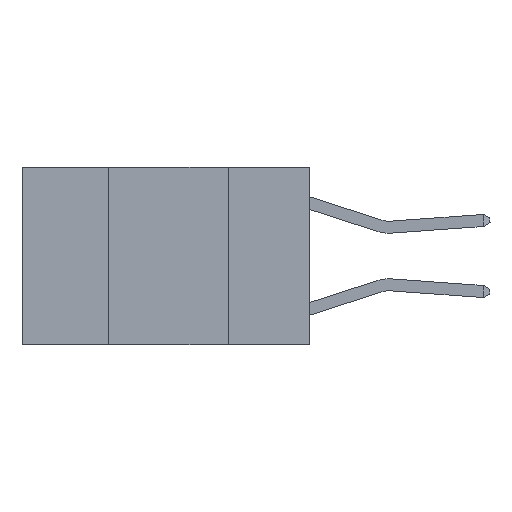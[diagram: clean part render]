
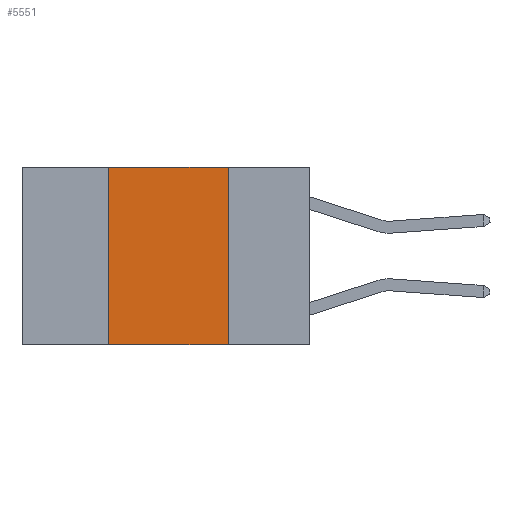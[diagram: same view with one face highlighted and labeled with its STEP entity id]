
A CAD part, left-side view. The second image highlights one B-rep face of the part: STEP entity #5551.
In plain terms, the highlighted planar face has unit normal (-1, 0, 0).
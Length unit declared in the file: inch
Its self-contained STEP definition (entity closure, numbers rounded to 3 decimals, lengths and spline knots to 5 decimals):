
#1247 = FACE_OUTER_BOUND ( 'NONE', #9727, .T. ) ;
#1549 = VERTEX_POINT ( 'NONE', #8327 ) ;
#1572 = CARTESIAN_POINT ( 'NONE',  ( 0., 0.6, 0. ) ) ;
#1805 = CARTESIAN_POINT ( 'NONE',  ( 0., 0.17, 0. ) ) ;
#2002 = CARTESIAN_POINT ( 'NONE',  ( 0., 0.6, 0. ) ) ;
#2233 = VECTOR ( 'NONE', #9315, 39.37008 ) ;
#2656 = DIRECTION ( 'NONE',  ( 0., -1., 0. ) ) ;
#2933 = EDGE_CURVE ( 'NONE', #13584, #8344, #10100, .T. ) ;
#3110 = DIRECTION ( 'NONE',  ( 0., 0., -1. ) ) ;
#3391 = DIRECTION ( 'NONE',  ( 0., 0., 1. ) ) ;
#3417 = ORIENTED_EDGE ( 'NONE', *, *, #9958, .F. ) ;
#3783 = VECTOR ( 'NONE', #3391, 39.37008 ) ;
#4291 = VECTOR ( 'NONE', #3110, 39.37008 ) ;
#4315 = VECTOR ( 'NONE', #2656, 39.37008 ) ;
#4911 = VERTEX_POINT ( 'NONE', #13449 ) ;
#5147 = ORIENTED_EDGE ( 'NONE', *, *, #2933, .F. ) ;
#5224 = EDGE_CURVE ( 'NONE', #1549, #4911, #11999, .T. ) ;
#5268 = PLANE ( 'NONE',  #9720 ) ;
#5498 = EDGE_CURVE ( 'NONE', #1549, #8344, #8744, .T. ) ;
#5551 = ADVANCED_FACE ( 'NONE', ( #1247 ), #5268, .F. ) ;
#6371 = DIRECTION ( 'NONE',  ( 0., 0., -1. ) ) ;
#6638 = CARTESIAN_POINT ( 'NONE',  ( 0., 0.42, 0. ) ) ;
#6971 = CARTESIAN_POINT ( 'NONE',  ( 0., 0.6, -0.37 ) ) ;
#7936 = LINE ( 'NONE', #1572, #4315 ) ;
#8327 = CARTESIAN_POINT ( 'NONE',  ( 0., 0.42, -0.37 ) ) ;
#8344 = VERTEX_POINT ( 'NONE', #12947 ) ;
#8744 = LINE ( 'NONE', #6971, #2233 ) ;
#9113 = ORIENTED_EDGE ( 'NONE', *, *, #5224, .F. ) ;
#9315 = DIRECTION ( 'NONE',  ( 0., -1., 0. ) ) ;
#9720 = AXIS2_PLACEMENT_3D ( 'NONE', #2002, #12731, #6371 ) ;
#9727 = EDGE_LOOP ( 'NONE', ( #5147, #3417, #9113, #11344 ) ) ;
#9958 = EDGE_CURVE ( 'NONE', #4911, #13584, #7936, .T. ) ;
#10100 = LINE ( 'NONE', #10690, #4291 ) ;
#10690 = CARTESIAN_POINT ( 'NONE',  ( 0., 0.17, 0. ) ) ;
#11344 = ORIENTED_EDGE ( 'NONE', *, *, #5498, .T. ) ;
#11999 = LINE ( 'NONE', #6638, #3783 ) ;
#12731 = DIRECTION ( 'NONE',  ( 1., 0., 0. ) ) ;
#12947 = CARTESIAN_POINT ( 'NONE',  ( 0., 0.17, -0.37 ) ) ;
#13449 = CARTESIAN_POINT ( 'NONE',  ( 0., 0.42, 0. ) ) ;
#13584 = VERTEX_POINT ( 'NONE', #1805 ) ;
